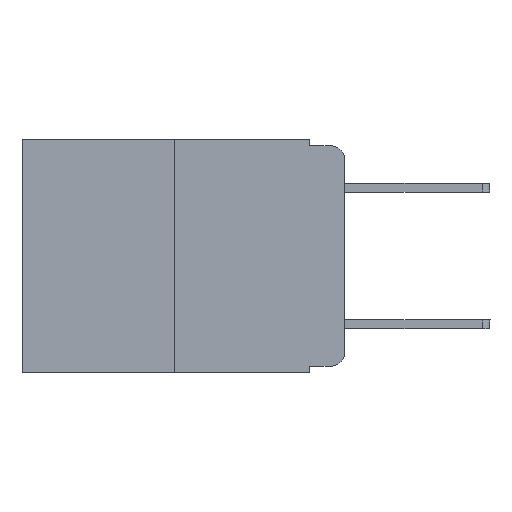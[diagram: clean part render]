
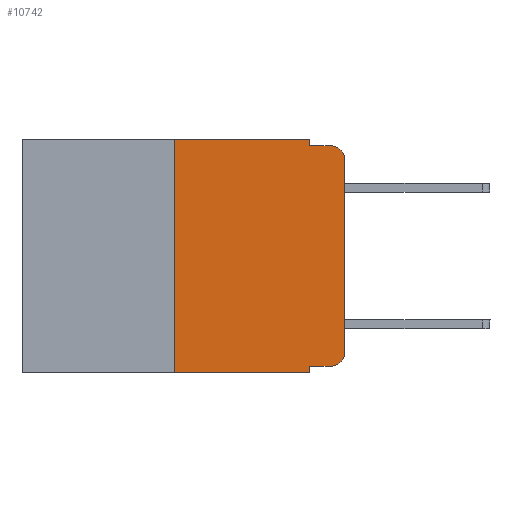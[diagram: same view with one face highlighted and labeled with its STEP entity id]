
A CAD part, left-side view. The second image highlights one B-rep face of the part: STEP entity #10742.
In plain terms, the highlighted planar face has unit normal (-1, 0, 0).
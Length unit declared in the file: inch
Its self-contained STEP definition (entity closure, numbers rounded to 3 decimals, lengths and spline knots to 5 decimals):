
#51 = ORIENTED_EDGE ( 'NONE', *, *, #4658, .F. ) ;
#330 = DIRECTION ( 'NONE',  ( 0., 0., 1. ) ) ;
#388 = VECTOR ( 'NONE', #4536, 39.37008 ) ;
#499 = CARTESIAN_POINT ( 'NONE',  ( 0., 0., -0.313 ) ) ;
#772 = AXIS2_PLACEMENT_3D ( 'NONE', #13761, #15005, #12529 ) ;
#807 = ORIENTED_EDGE ( 'NONE', *, *, #14657, .F. ) ;
#825 = EDGE_CURVE ( 'NONE', #15393, #10233, #14973, .T. ) ;
#1434 = CARTESIAN_POINT ( 'NONE',  ( 0., 0.051, -0.343 ) ) ;
#1695 = DIRECTION ( 'NONE',  ( 0., 0., -1. ) ) ;
#1834 = CARTESIAN_POINT ( 'NONE',  ( 0., 0.473, 0. ) ) ;
#1933 = VECTOR ( 'NONE', #10037, 39.37008 ) ;
#2004 = LINE ( 'NONE', #1834, #15493 ) ;
#2227 = CARTESIAN_POINT ( 'NONE',  ( 0., 0.473, -0.343 ) ) ;
#2282 = ORIENTED_EDGE ( 'NONE', *, *, #11174, .T. ) ;
#2433 = CARTESIAN_POINT ( 'NONE',  ( 0., 0.25, -0.343 ) ) ;
#3014 = PLANE ( 'NONE',  #6306 ) ;
#3859 = CARTESIAN_POINT ( 'NONE',  ( 0., 0.051, -0.333 ) ) ;
#4085 = DIRECTION ( 'NONE',  ( 1., 0., 0. ) ) ;
#4236 = VECTOR ( 'NONE', #15738, 39.37008 ) ;
#4348 = CARTESIAN_POINT ( 'NONE',  ( 0., 0.051, 0. ) ) ;
#4349 = CARTESIAN_POINT ( 'NONE',  ( 0., 0.02, -0.01 ) ) ;
#4485 = ORIENTED_EDGE ( 'NONE', *, *, #10179, .T. ) ;
#4536 = DIRECTION ( 'NONE',  ( 0., 0., 1. ) ) ;
#4581 = EDGE_CURVE ( 'NONE', #12394, #6465, #9059, .T. ) ;
#4658 = EDGE_CURVE ( 'NONE', #9495, #7444, #9387, .T. ) ;
#4740 = EDGE_CURVE ( 'NONE', #11083, #9334, #6901, .T. ) ;
#5009 = CARTESIAN_POINT ( 'NONE',  ( 0., 0.051, -0.01 ) ) ;
#5271 = LINE ( 'NONE', #3859, #15414 ) ;
#5613 = ORIENTED_EDGE ( 'NONE', *, *, #9423, .F. ) ;
#5799 = DIRECTION ( 'NONE',  ( 0., -1., 0. ) ) ;
#5840 = CARTESIAN_POINT ( 'NONE',  ( 0., 0.02, -0.333 ) ) ;
#6306 = AXIS2_PLACEMENT_3D ( 'NONE', #7802, #4085, #1695 ) ;
#6465 = VERTEX_POINT ( 'NONE', #7296 ) ;
#6901 = LINE ( 'NONE', #10698, #4236 ) ;
#7178 = CARTESIAN_POINT ( 'NONE',  ( 0., 0.051, -0.01 ) ) ;
#7296 = CARTESIAN_POINT ( 'NONE',  ( 0., 0.25, 0. ) ) ;
#7444 = VERTEX_POINT ( 'NONE', #7178 ) ;
#7539 = VERTEX_POINT ( 'NONE', #499 ) ;
#7656 = DIRECTION ( 'NONE',  ( 0., -1., 0. ) ) ;
#7697 = VERTEX_POINT ( 'NONE', #5840 ) ;
#7802 = CARTESIAN_POINT ( 'NONE',  ( 0., 0.473, 0. ) ) ;
#8058 = DIRECTION ( 'NONE',  ( 0., 0., -1. ) ) ;
#8064 = ORIENTED_EDGE ( 'NONE', *, *, #11819, .T. ) ;
#8715 = LINE ( 'NONE', #5009, #1933 ) ;
#9059 = LINE ( 'NONE', #12675, #12389 ) ;
#9177 = CARTESIAN_POINT ( 'NONE',  ( 0., 0., 0. ) ) ;
#9334 = VERTEX_POINT ( 'NONE', #1434 ) ;
#9387 = LINE ( 'NONE', #4348, #10564 ) ;
#9423 = EDGE_CURVE ( 'NONE', #6465, #9495, #2004, .T. ) ;
#9495 = VERTEX_POINT ( 'NONE', #15693 ) ;
#9711 = CARTESIAN_POINT ( 'NONE',  ( 0., 0.02, -0.313 ) ) ;
#10037 = DIRECTION ( 'NONE',  ( 0., -1., 0. ) ) ;
#10179 = EDGE_CURVE ( 'NONE', #11083, #7697, #5271, .T. ) ;
#10233 = VERTEX_POINT ( 'NONE', #4349 ) ;
#10539 = ORIENTED_EDGE ( 'NONE', *, *, #4740, .F. ) ;
#10564 = VECTOR ( 'NONE', #8058, 39.37008 ) ;
#10698 = CARTESIAN_POINT ( 'NONE',  ( 0., 0.051, 0. ) ) ;
#10742 = ADVANCED_FACE ( 'NONE', ( #11754 ), #3014, .F. ) ;
#11083 = VERTEX_POINT ( 'NONE', #16213 ) ;
#11132 = VECTOR ( 'NONE', #15930, 39.37008 ) ;
#11174 = EDGE_CURVE ( 'NONE', #7539, #15393, #11489, .T. ) ;
#11489 = LINE ( 'NONE', #9177, #388 ) ;
#11754 = FACE_OUTER_BOUND ( 'NONE', #12284, .T. ) ;
#11819 = EDGE_CURVE ( 'NONE', #7697, #7539, #13856, .T. ) ;
#11899 = CARTESIAN_POINT ( 'NONE',  ( 0., 0., -0.03 ) ) ;
#12284 = EDGE_LOOP ( 'NONE', ( #2282, #15525, #807, #51, #5613, #12741, #15014, #10539, #4485, #8064 ) ) ;
#12309 = AXIS2_PLACEMENT_3D ( 'NONE', #9711, #16146, #13494 ) ;
#12389 = VECTOR ( 'NONE', #330, 39.37008 ) ;
#12394 = VERTEX_POINT ( 'NONE', #2433 ) ;
#12529 = DIRECTION ( 'NONE',  ( 0., 0., -1. ) ) ;
#12675 = CARTESIAN_POINT ( 'NONE',  ( 0., 0.25, 0. ) ) ;
#12741 = ORIENTED_EDGE ( 'NONE', *, *, #4581, .F. ) ;
#13437 = LINE ( 'NONE', #2227, #11132 ) ;
#13494 = DIRECTION ( 'NONE',  ( 0., 0., -1. ) ) ;
#13761 = CARTESIAN_POINT ( 'NONE',  ( 0., 0.02, -0.03 ) ) ;
#13856 = CIRCLE ( 'NONE', #12309, 0.02 ) ;
#13858 = EDGE_CURVE ( 'NONE', #12394, #9334, #13437, .T. ) ;
#14657 = EDGE_CURVE ( 'NONE', #7444, #10233, #8715, .T. ) ;
#14973 = CIRCLE ( 'NONE', #772, 0.02 ) ;
#15005 = DIRECTION ( 'NONE',  ( -1., 0., 0. ) ) ;
#15014 = ORIENTED_EDGE ( 'NONE', *, *, #13858, .T. ) ;
#15393 = VERTEX_POINT ( 'NONE', #11899 ) ;
#15414 = VECTOR ( 'NONE', #7656, 39.37008 ) ;
#15493 = VECTOR ( 'NONE', #5799, 39.37008 ) ;
#15525 = ORIENTED_EDGE ( 'NONE', *, *, #825, .T. ) ;
#15693 = CARTESIAN_POINT ( 'NONE',  ( 0., 0.051, 0. ) ) ;
#15738 = DIRECTION ( 'NONE',  ( 0., 0., -1. ) ) ;
#15930 = DIRECTION ( 'NONE',  ( 0., -1., 0. ) ) ;
#16146 = DIRECTION ( 'NONE',  ( -1., 0., 0. ) ) ;
#16213 = CARTESIAN_POINT ( 'NONE',  ( 0., 0.051, -0.333 ) ) ;
